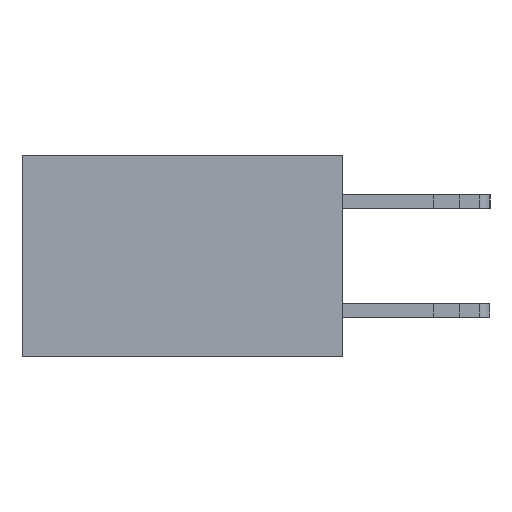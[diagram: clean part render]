
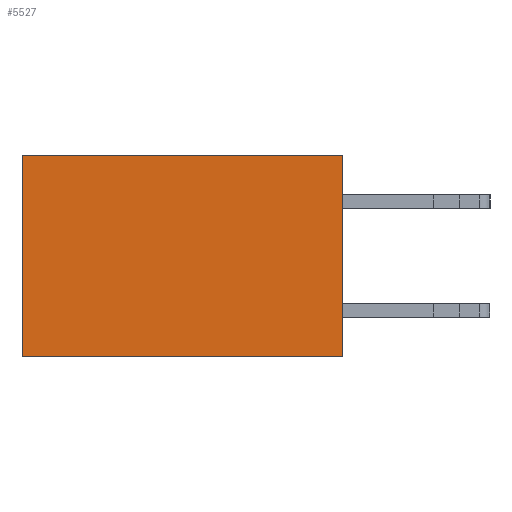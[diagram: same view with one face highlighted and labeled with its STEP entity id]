
A CAD part, left-side view. The second image highlights one B-rep face of the part: STEP entity #5527.
In plain terms, the highlighted planar face has unit normal (-1, 0, 0).
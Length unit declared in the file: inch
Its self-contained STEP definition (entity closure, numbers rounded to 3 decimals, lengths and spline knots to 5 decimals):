
#937 = LINE ( 'NONE', #10240, #7260 ) ;
#1672 = ORIENTED_EDGE ( 'NONE', *, *, #2123, .F. ) ;
#2123 = EDGE_CURVE ( 'NONE', #5809, #11150, #8298, .T. ) ;
#3125 = LINE ( 'NONE', #9607, #9435 ) ;
#3770 = VERTEX_POINT ( 'NONE', #15684 ) ;
#4951 = VECTOR ( 'NONE', #14511, 39.37008 ) ;
#5498 = CARTESIAN_POINT ( 'NONE',  ( 0.277, 0.59, -0.37 ) ) ;
#5527 = ADVANCED_FACE ( 'NONE', ( #14780 ), #15139, .F. ) ;
#5633 = ORIENTED_EDGE ( 'NONE', *, *, #10350, .T. ) ;
#5809 = VERTEX_POINT ( 'NONE', #12708 ) ;
#6096 = CARTESIAN_POINT ( 'NONE',  ( 0.277, 0.59, 0. ) ) ;
#6097 = EDGE_CURVE ( 'NONE', #11150, #3770, #937, .T. ) ;
#6153 = EDGE_CURVE ( 'NONE', #5809, #7461, #3125, .T. ) ;
#7133 = EDGE_LOOP ( 'NONE', ( #5633, #10220, #1672, #13219 ) ) ;
#7221 = AXIS2_PLACEMENT_3D ( 'NONE', #15164, #15114, #15096 ) ;
#7260 = VECTOR ( 'NONE', #10164, 39.37008 ) ;
#7461 = VERTEX_POINT ( 'NONE', #6096 ) ;
#8298 = LINE ( 'NONE', #14156, #4951 ) ;
#9422 = CARTESIAN_POINT ( 'NONE',  ( 0.277, 0., -0.37 ) ) ;
#9435 = VECTOR ( 'NONE', #9546, 39.37008 ) ;
#9546 = DIRECTION ( 'NONE',  ( 0., 1., 0. ) ) ;
#9607 = CARTESIAN_POINT ( 'NONE',  ( 0.277, 0., 0. ) ) ;
#9723 = VECTOR ( 'NONE', #15546, 39.37008 ) ;
#10164 = DIRECTION ( 'NONE',  ( 0., 1., 0. ) ) ;
#10220 = ORIENTED_EDGE ( 'NONE', *, *, #6097, .F. ) ;
#10240 = CARTESIAN_POINT ( 'NONE',  ( 0.277, 0., -0.37 ) ) ;
#10350 = EDGE_CURVE ( 'NONE', #7461, #3770, #11864, .T. ) ;
#11150 = VERTEX_POINT ( 'NONE', #9422 ) ;
#11864 = LINE ( 'NONE', #5498, #9723 ) ;
#12708 = CARTESIAN_POINT ( 'NONE',  ( 0.277, 0., 0. ) ) ;
#13219 = ORIENTED_EDGE ( 'NONE', *, *, #6153, .T. ) ;
#14156 = CARTESIAN_POINT ( 'NONE',  ( 0.277, 0., -0.37 ) ) ;
#14511 = DIRECTION ( 'NONE',  ( 0., 0., -1. ) ) ;
#14780 = FACE_OUTER_BOUND ( 'NONE', #7133, .T. ) ;
#15096 = DIRECTION ( 'NONE',  ( 0., 0., -1. ) ) ;
#15114 = DIRECTION ( 'NONE',  ( 1., 0., 0. ) ) ;
#15139 = PLANE ( 'NONE',  #7221 ) ;
#15164 = CARTESIAN_POINT ( 'NONE',  ( 0.277, 0., -0.37 ) ) ;
#15546 = DIRECTION ( 'NONE',  ( 0., 0., -1. ) ) ;
#15684 = CARTESIAN_POINT ( 'NONE',  ( 0.277, 0.59, -0.37 ) ) ;
